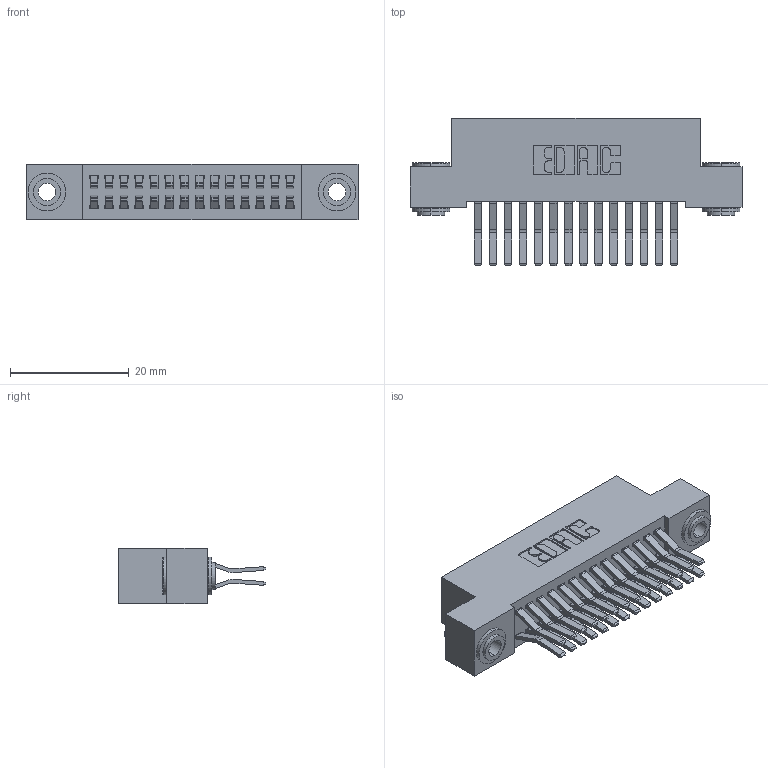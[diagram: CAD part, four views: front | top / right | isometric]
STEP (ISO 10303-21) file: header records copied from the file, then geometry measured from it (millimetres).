
FILE_DESCRIPTION (( 'STEP AP203' ), '1' );
FILE_NAME ('342-028-560-203.STEP', '2018-08-11T14:37:49', ( '' ), ( '' ), 'SwSTEP 2.0', 'SolidWorks 2016', '' );
FILE_SCHEMA (( 'CONFIG_CONTROL_DESIGN' ));
Length unit declared in the file: inch
Products named in the file (4): 342-250-002_345-250-002-102; 342-028-560-203; 342 Part_.156 TH; 345-292-001_560 Tail
Assembly tree (31 placements, depth 2):
  342-028-560-203
    342 Part_.156 TH
    345-292-001_560 Tail  x28
    342-250-002_345-250-002-102  x2
Bounding box: 55.88 x 24.78 x 9.4 mm (x, y, z)
Volume: 5094.9 mm3; surface area: 8258.2 mm2
Topology: 31 solids, 31 shells, 1660 faces, 4883 edges, 3214 vertices
Faces by surface type: plane 1084, cylinder 568, cone 8
Entity records: 13234 total; most frequent: CARTESIAN_POINT 2201, ORIENTED_EDGE 2130, DIRECTION 1967, EDGE_CURVE 1065, LINE 909, VECTOR 909, VERTEX_POINT 706, AXIS2_PLACEMENT_3D 529
